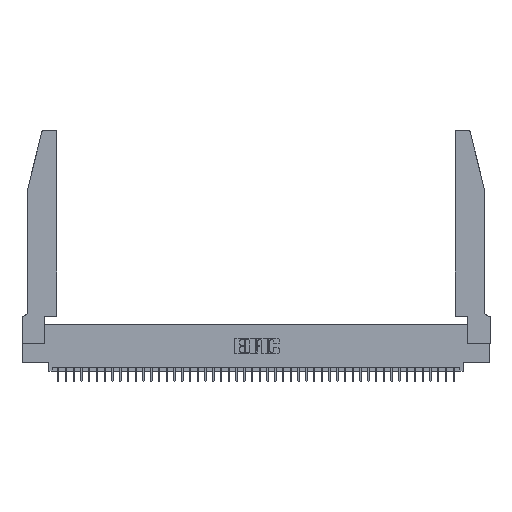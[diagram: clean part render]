
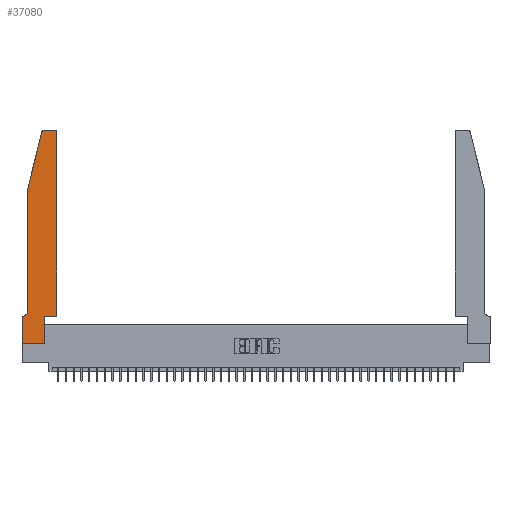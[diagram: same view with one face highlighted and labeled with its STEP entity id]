
A CAD part, top view. The second image highlights one B-rep face of the part: STEP entity #37080.
In plain terms, the highlighted planar face has unit normal (0, 0, 1).
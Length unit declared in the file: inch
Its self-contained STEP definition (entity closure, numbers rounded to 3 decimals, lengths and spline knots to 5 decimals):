
#513 = CARTESIAN_POINT ( 'NONE',  ( 0.2605, 2.75, 0.37 ) ) ;
#1244 = EDGE_CURVE ( 'NONE', #17616, #9385, #18555, .T. ) ;
#1572 = ORIENTED_EDGE ( 'NONE', *, *, #37156, .T. ) ;
#2273 = CARTESIAN_POINT ( 'NONE',  ( 0.4205, 2.72, 0.37 ) ) ;
#3293 = CIRCLE ( 'NONE', #4740, 0.07 ) ;
#3445 = LINE ( 'NONE', #13335, #20149 ) ;
#3551 = CARTESIAN_POINT ( 'NONE',  ( 0.284, 2.75, 0.37 ) ) ;
#4313 = ORIENTED_EDGE ( 'NONE', *, *, #18824, .T. ) ;
#4647 = DIRECTION ( 'NONE',  ( 0., -1., 0. ) ) ;
#4740 = AXIS2_PLACEMENT_3D ( 'NONE', #20348, #20118, #40648 ) ;
#6408 = VERTEX_POINT ( 'NONE', #39119 ) ;
#7652 = AXIS2_PLACEMENT_3D ( 'NONE', #42327, #22035, #21359 ) ;
#8244 = ORIENTED_EDGE ( 'NONE', *, *, #28612, .T. ) ;
#8456 = CARTESIAN_POINT ( 'NONE',  ( 0., 0., 0.37 ) ) ;
#9385 = VERTEX_POINT ( 'NONE', #41813 ) ;
#9704 = DIRECTION ( 'NONE',  ( 1., 0., 0. ) ) ;
#9809 = CIRCLE ( 'NONE', #7652, 0.03 ) ;
#9850 = EDGE_CURVE ( 'NONE', #6408, #19069, #30779, .T. ) ;
#9943 = AXIS2_PLACEMENT_3D ( 'NONE', #2273, #12406, #36657 ) ;
#10278 = DIRECTION ( 'NONE',  ( 0., -1., 0. ) ) ;
#10613 = EDGE_CURVE ( 'NONE', #19069, #36419, #3445, .T. ) ;
#10685 = CARTESIAN_POINT ( 'NONE',  ( 0., 0.35, 0.37 ) ) ;
#11060 = LINE ( 'NONE', #34198, #24939 ) ;
#11977 = LINE ( 'NONE', #36444, #40123 ) ;
#12078 = AXIS2_PLACEMENT_3D ( 'NONE', #10685, #28865, #42560 ) ;
#12406 = DIRECTION ( 'NONE',  ( 0., 0., 1. ) ) ;
#12896 = CARTESIAN_POINT ( 'NONE',  ( 0.2865, 0., 0.37 ) ) ;
#13228 = CARTESIAN_POINT ( 'NONE',  ( 0.4505, 0.35, 0.37 ) ) ;
#13285 = LINE ( 'NONE', #8456, #13834 ) ;
#13335 = CARTESIAN_POINT ( 'NONE',  ( 0.4505, 0.35, 0.37 ) ) ;
#13834 = VECTOR ( 'NONE', #9704, 39.37008 ) ;
#14462 = CARTESIAN_POINT ( 'NONE',  ( 0.0755, 2., 0.37 ) ) ;
#15164 = ORIENTED_EDGE ( 'NONE', *, *, #37118, .T. ) ;
#15248 = VERTEX_POINT ( 'NONE', #3551 ) ;
#17464 = CARTESIAN_POINT ( 'NONE',  ( 0.4505, 0.35, 0.37 ) ) ;
#17535 = CARTESIAN_POINT ( 'NONE',  ( 0.0755, 2., 0.37 ) ) ;
#17616 = VERTEX_POINT ( 'NONE', #14462 ) ;
#18225 = FACE_OUTER_BOUND ( 'NONE', #34133, .T. ) ;
#18540 = VERTEX_POINT ( 'NONE', #29106 ) ;
#18555 = LINE ( 'NONE', #28979, #20496 ) ;
#18824 = EDGE_CURVE ( 'NONE', #42031, #6408, #11060, .T. ) ;
#18901 = EDGE_CURVE ( 'NONE', #28673, #17616, #34636, .T. ) ;
#19069 = VERTEX_POINT ( 'NONE', #13228 ) ;
#19135 = DIRECTION ( 'NONE',  ( 1., 0., 0. ) ) ;
#19994 = ORIENTED_EDGE ( 'NONE', *, *, #26403, .T. ) ;
#20118 = DIRECTION ( 'NONE',  ( 0., 0., -1. ) ) ;
#20149 = VECTOR ( 'NONE', #33798, 39.37008 ) ;
#20348 = CARTESIAN_POINT ( 'NONE',  ( 0.0055, 0.42, 0.37 ) ) ;
#20496 = VECTOR ( 'NONE', #4647, 39.37008 ) ;
#20934 = DIRECTION ( 'NONE',  ( -1., 0., 0. ) ) ;
#21359 = DIRECTION ( 'NONE',  ( 1., 0., 0. ) ) ;
#21851 = ORIENTED_EDGE ( 'NONE', *, *, #1244, .T. ) ;
#22035 = DIRECTION ( 'NONE',  ( 0., 0., 1. ) ) ;
#23156 = ORIENTED_EDGE ( 'NONE', *, *, #18901, .T. ) ;
#23530 = CIRCLE ( 'NONE', #9943, 0.03 ) ;
#23685 = VERTEX_POINT ( 'NONE', #36450 ) ;
#24939 = VECTOR ( 'NONE', #31726, 39.37008 ) ;
#25037 = CARTESIAN_POINT ( 'NONE',  ( 0.25487, 2.72718, 0.37 ) ) ;
#25214 = DIRECTION ( 'NONE',  ( -0.239, -0.971, 0. ) ) ;
#26403 = EDGE_CURVE ( 'NONE', #18540, #42031, #13285, .T. ) ;
#26981 = ORIENTED_EDGE ( 'NONE', *, *, #10613, .T. ) ;
#28612 = EDGE_CURVE ( 'NONE', #23685, #15248, #31999, .T. ) ;
#28673 = VERTEX_POINT ( 'NONE', #25037 ) ;
#28865 = DIRECTION ( 'NONE',  ( 0., 0., 1. ) ) ;
#28979 = CARTESIAN_POINT ( 'NONE',  ( 0.0755, 2., 0.37 ) ) ;
#29103 = ORIENTED_EDGE ( 'NONE', *, *, #36471, .T. ) ;
#29106 = CARTESIAN_POINT ( 'NONE',  ( 0., 0., 0.37 ) ) ;
#29107 = VECTOR ( 'NONE', #20934, 39.37008 ) ;
#29730 = DIRECTION ( 'NONE',  ( -1., 0., 0. ) ) ;
#30096 = CARTESIAN_POINT ( 'NONE',  ( 0., 0., 0.37 ) ) ;
#30530 = EDGE_CURVE ( 'NONE', #9385, #42414, #3293, .T. ) ;
#30655 = EDGE_CURVE ( 'NONE', #15248, #28673, #9809, .T. ) ;
#30779 = LINE ( 'NONE', #17464, #33110 ) ;
#31726 = DIRECTION ( 'NONE',  ( 0., 1., 0. ) ) ;
#31999 = LINE ( 'NONE', #513, #29107 ) ;
#33110 = VECTOR ( 'NONE', #19135, 39.37008 ) ;
#33665 = LINE ( 'NONE', #30096, #40182 ) ;
#33798 = DIRECTION ( 'NONE',  ( 0., 1., 0. ) ) ;
#34133 = EDGE_LOOP ( 'NONE', ( #8244, #41703, #23156, #21851, #37764, #1572, #29103, #19994, #4313, #37843, #26981, #15164 ) ) ;
#34198 = CARTESIAN_POINT ( 'NONE',  ( 0.2865, 0.35, 0.37 ) ) ;
#34287 = CARTESIAN_POINT ( 'NONE',  ( 0., 0.35, 0.37 ) ) ;
#34636 = LINE ( 'NONE', #17535, #41439 ) ;
#36419 = VERTEX_POINT ( 'NONE', #37468 ) ;
#36444 = CARTESIAN_POINT ( 'NONE',  ( 0.0755, 0.35, 0.37 ) ) ;
#36450 = CARTESIAN_POINT ( 'NONE',  ( 0.4205, 2.75, 0.37 ) ) ;
#36471 = EDGE_CURVE ( 'NONE', #38284, #18540, #33665, .T. ) ;
#36657 = DIRECTION ( 'NONE',  ( 1., 0., 0. ) ) ;
#37080 = ADVANCED_FACE ( 'NONE', ( #18225 ), #37640, .T. ) ;
#37118 = EDGE_CURVE ( 'NONE', #36419, #23685, #23530, .T. ) ;
#37156 = EDGE_CURVE ( 'NONE', #42414, #38284, #11977, .T. ) ;
#37468 = CARTESIAN_POINT ( 'NONE',  ( 0.4505, 2.72, 0.37 ) ) ;
#37640 = PLANE ( 'NONE',  #12078 ) ;
#37764 = ORIENTED_EDGE ( 'NONE', *, *, #30530, .T. ) ;
#37843 = ORIENTED_EDGE ( 'NONE', *, *, #9850, .T. ) ;
#38284 = VERTEX_POINT ( 'NONE', #34287 ) ;
#39119 = CARTESIAN_POINT ( 'NONE',  ( 0.2865, 0.35, 0.37 ) ) ;
#40069 = CARTESIAN_POINT ( 'NONE',  ( 0.0055, 0.35, 0.37 ) ) ;
#40123 = VECTOR ( 'NONE', #29730, 39.37008 ) ;
#40182 = VECTOR ( 'NONE', #10278, 39.37008 ) ;
#40648 = DIRECTION ( 'NONE',  ( -1., 0., 0. ) ) ;
#41439 = VECTOR ( 'NONE', #25214, 39.37008 ) ;
#41703 = ORIENTED_EDGE ( 'NONE', *, *, #30655, .T. ) ;
#41813 = CARTESIAN_POINT ( 'NONE',  ( 0.0755, 0.42, 0.37 ) ) ;
#42031 = VERTEX_POINT ( 'NONE', #12896 ) ;
#42327 = CARTESIAN_POINT ( 'NONE',  ( 0.284, 2.72, 0.37 ) ) ;
#42414 = VERTEX_POINT ( 'NONE', #40069 ) ;
#42560 = DIRECTION ( 'NONE',  ( 1., 0., 0. ) ) ;
